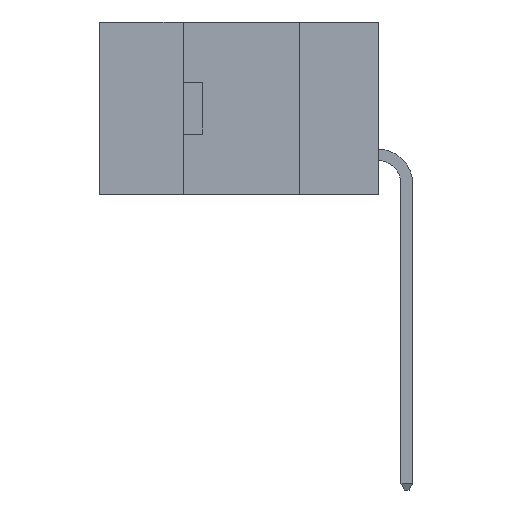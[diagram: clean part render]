
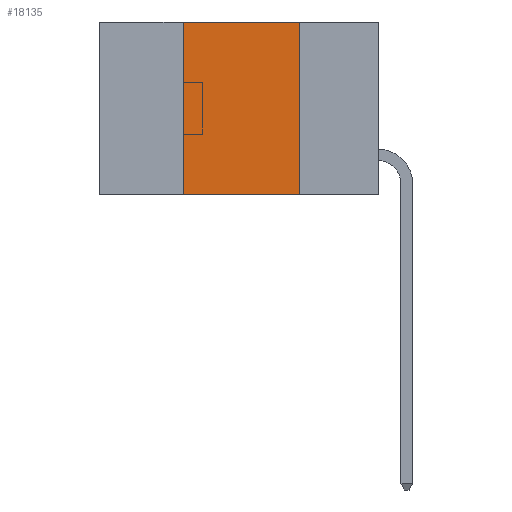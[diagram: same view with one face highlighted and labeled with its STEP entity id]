
A CAD part, left-side view. The second image highlights one B-rep face of the part: STEP entity #18135.
In plain terms, the highlighted planar face has unit normal (-1, 0, 0).
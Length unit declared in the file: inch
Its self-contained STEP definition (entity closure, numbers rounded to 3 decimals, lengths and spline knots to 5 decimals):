
#311 = DIRECTION ( 'NONE',  ( 0., -1., 0. ) ) ;
#2658 = FACE_OUTER_BOUND ( 'NONE', #17852, .T. ) ;
#3308 = CARTESIAN_POINT ( 'NONE',  ( 0., 0.42, -0.37 ) ) ;
#4660 = VECTOR ( 'NONE', #311, 39.37008 ) ;
#4946 = DIRECTION ( 'NONE',  ( 0., -1., 0. ) ) ;
#5005 = EDGE_CURVE ( 'NONE', #8163, #7396, #16904, .T. ) ;
#6810 = CARTESIAN_POINT ( 'NONE',  ( 0., 0.17, -0.37 ) ) ;
#7026 = CARTESIAN_POINT ( 'NONE',  ( 0., 0.6, 0. ) ) ;
#7396 = VERTEX_POINT ( 'NONE', #19045 ) ;
#7651 = VECTOR ( 'NONE', #16200, 39.37008 ) ;
#8163 = VERTEX_POINT ( 'NONE', #8525 ) ;
#8525 = CARTESIAN_POINT ( 'NONE',  ( 0., 0.42, 0. ) ) ;
#9191 = DIRECTION ( 'NONE',  ( 1., 0., 0. ) ) ;
#9244 = CARTESIAN_POINT ( 'NONE',  ( 0., 0.42, -0.37 ) ) ;
#10979 = VERTEX_POINT ( 'NONE', #9244 ) ;
#11230 = VECTOR ( 'NONE', #4946, 39.37008 ) ;
#13243 = EDGE_CURVE ( 'NONE', #10979, #8163, #14063, .T. ) ;
#14063 = LINE ( 'NONE', #3308, #7651 ) ;
#14287 = ORIENTED_EDGE ( 'NONE', *, *, #5005, .F. ) ;
#14483 = ORIENTED_EDGE ( 'NONE', *, *, #18046, .T. ) ;
#15114 = VERTEX_POINT ( 'NONE', #26030 ) ;
#15778 = AXIS2_PLACEMENT_3D ( 'NONE', #7026, #9191, #24065 ) ;
#15976 = VECTOR ( 'NONE', #17620, 39.37008 ) ;
#16200 = DIRECTION ( 'NONE',  ( 0., 0., 1. ) ) ;
#16904 = LINE ( 'NONE', #26136, #11230 ) ;
#17459 = CARTESIAN_POINT ( 'NONE',  ( 0., 0.6, -0.37 ) ) ;
#17620 = DIRECTION ( 'NONE',  ( 0., 0., -1. ) ) ;
#17852 = EDGE_LOOP ( 'NONE', ( #25162, #14287, #25218, #14483 ) ) ;
#18046 = EDGE_CURVE ( 'NONE', #10979, #15114, #21732, .T. ) ;
#18135 = ADVANCED_FACE ( 'NONE', ( #2658 ), #21965, .F. ) ;
#19045 = CARTESIAN_POINT ( 'NONE',  ( 0., 0.17, 0. ) ) ;
#21567 = LINE ( 'NONE', #6810, #15976 ) ;
#21732 = LINE ( 'NONE', #17459, #4660 ) ;
#21965 = PLANE ( 'NONE',  #15778 ) ;
#23948 = EDGE_CURVE ( 'NONE', #7396, #15114, #21567, .T. ) ;
#24065 = DIRECTION ( 'NONE',  ( 0., 0., -1. ) ) ;
#25162 = ORIENTED_EDGE ( 'NONE', *, *, #23948, .F. ) ;
#25218 = ORIENTED_EDGE ( 'NONE', *, *, #13243, .F. ) ;
#26030 = CARTESIAN_POINT ( 'NONE',  ( 0., 0.17, -0.37 ) ) ;
#26136 = CARTESIAN_POINT ( 'NONE',  ( 0., 0.6, 0. ) ) ;
